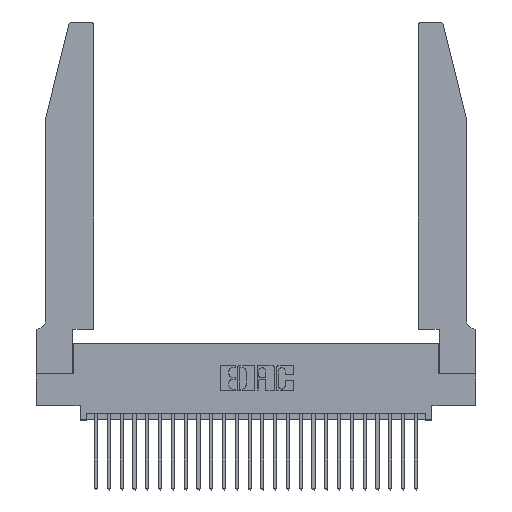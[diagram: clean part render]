
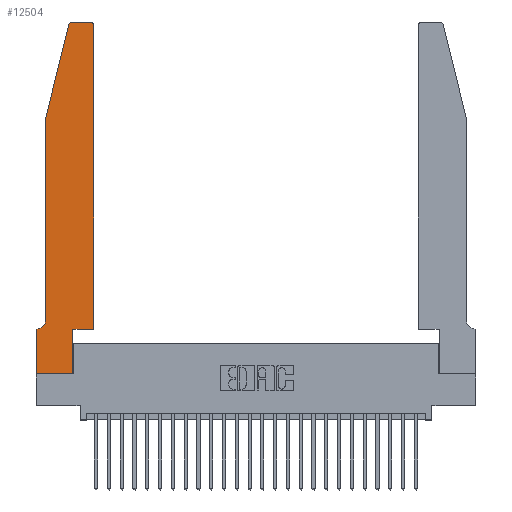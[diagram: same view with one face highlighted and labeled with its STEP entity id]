
A CAD part, top view. The second image highlights one B-rep face of the part: STEP entity #12504.
In plain terms, the highlighted planar face has unit normal (0, 0, 1).
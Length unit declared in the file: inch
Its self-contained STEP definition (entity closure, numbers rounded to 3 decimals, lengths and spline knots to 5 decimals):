
#205 = DIRECTION ( 'NONE',  ( 1., 0., 0. ) ) ;
#314 = ORIENTED_EDGE ( 'NONE', *, *, #13325, .T. ) ;
#342 = CARTESIAN_POINT ( 'NONE',  ( 0.284, 2.75, 0.37 ) ) ;
#738 = DIRECTION ( 'NONE',  ( 1., 0., 0. ) ) ;
#1029 = CARTESIAN_POINT ( 'NONE',  ( 0.25487, 2.72718, 0.37 ) ) ;
#1056 = CARTESIAN_POINT ( 'NONE',  ( 0.4205, 2.72, 0.37 ) ) ;
#1068 = VECTOR ( 'NONE', #16435, 39.37008 ) ;
#1119 = EDGE_CURVE ( 'NONE', #14258, #14778, #4081, .T. ) ;
#1410 = CARTESIAN_POINT ( 'NONE',  ( 0., 0., 0.37 ) ) ;
#1441 = LINE ( 'NONE', #9090, #6579 ) ;
#1597 = VECTOR ( 'NONE', #4198, 39.37008 ) ;
#1610 = LINE ( 'NONE', #23052, #12363 ) ;
#2075 = DIRECTION ( 'NONE',  ( 1., 0., 0. ) ) ;
#3099 = AXIS2_PLACEMENT_3D ( 'NONE', #27388, #14847, #2075 ) ;
#3253 = DIRECTION ( 'NONE',  ( 1., 0., 0. ) ) ;
#3386 = VECTOR ( 'NONE', #16997, 39.37008 ) ;
#3695 = VERTEX_POINT ( 'NONE', #342 ) ;
#3972 = CARTESIAN_POINT ( 'NONE',  ( 0.4505, 0.35, 0.37 ) ) ;
#4081 = LINE ( 'NONE', #23432, #3386 ) ;
#4198 = DIRECTION ( 'NONE',  ( -1., 0., 0. ) ) ;
#4357 = VERTEX_POINT ( 'NONE', #17513 ) ;
#4765 = VECTOR ( 'NONE', #12506, 39.37008 ) ;
#5065 = DIRECTION ( 'NONE',  ( 0., 0., -1. ) ) ;
#5778 = VECTOR ( 'NONE', #10602, 39.37008 ) ;
#5875 = FACE_OUTER_BOUND ( 'NONE', #19694, .T. ) ;
#5884 = ORIENTED_EDGE ( 'NONE', *, *, #19129, .T. ) ;
#6172 = EDGE_CURVE ( 'NONE', #13839, #14258, #1441, .T. ) ;
#6208 = AXIS2_PLACEMENT_3D ( 'NONE', #1056, #16011, #3253 ) ;
#6437 = CARTESIAN_POINT ( 'NONE',  ( 0.2865, 0.35, 0.37 ) ) ;
#6579 = VECTOR ( 'NONE', #15410, 39.37008 ) ;
#6647 = DIRECTION ( 'NONE',  ( 0., 1., 0. ) ) ;
#6660 = CARTESIAN_POINT ( 'NONE',  ( 0.0755, 2., 0.37 ) ) ;
#6893 = LINE ( 'NONE', #1410, #1068 ) ;
#7724 = ORIENTED_EDGE ( 'NONE', *, *, #6172, .T. ) ;
#8685 = EDGE_CURVE ( 'NONE', #4357, #13031, #1610, .T. ) ;
#9027 = LINE ( 'NONE', #3972, #19494 ) ;
#9090 = CARTESIAN_POINT ( 'NONE',  ( 0.0755, 2., 0.37 ) ) ;
#9771 = EDGE_CURVE ( 'NONE', #3695, #13839, #20169, .T. ) ;
#9810 = ORIENTED_EDGE ( 'NONE', *, *, #26122, .T. ) ;
#10602 = DIRECTION ( 'NONE',  ( -1., 0., 0. ) ) ;
#10643 = CARTESIAN_POINT ( 'NONE',  ( 0., 0.35, 0.37 ) ) ;
#11030 = ORIENTED_EDGE ( 'NONE', *, *, #17506, .T. ) ;
#11742 = EDGE_CURVE ( 'NONE', #14778, #12065, #23650, .T. ) ;
#12009 = EDGE_CURVE ( 'NONE', #13031, #23564, #17102, .T. ) ;
#12065 = VERTEX_POINT ( 'NONE', #17816 ) ;
#12188 = VECTOR ( 'NONE', #738, 39.37008 ) ;
#12207 = EDGE_CURVE ( 'NONE', #18627, #4357, #6893, .T. ) ;
#12313 = CARTESIAN_POINT ( 'NONE',  ( 0.4205, 2.75, 0.37 ) ) ;
#12363 = VECTOR ( 'NONE', #25150, 39.37008 ) ;
#12504 = ADVANCED_FACE ( 'NONE', ( #5875 ), #17228, .T. ) ;
#12506 = DIRECTION ( 'NONE',  ( 0., -1., 0. ) ) ;
#12954 = ORIENTED_EDGE ( 'NONE', *, *, #1119, .T. ) ;
#13031 = VERTEX_POINT ( 'NONE', #6437 ) ;
#13033 = CARTESIAN_POINT ( 'NONE',  ( 0., 0., 0.37 ) ) ;
#13067 = AXIS2_PLACEMENT_3D ( 'NONE', #25637, #13104, #205 ) ;
#13104 = DIRECTION ( 'NONE',  ( 0., 0., 1. ) ) ;
#13325 = EDGE_CURVE ( 'NONE', #18526, #26682, #24911, .T. ) ;
#13839 = VERTEX_POINT ( 'NONE', #1029 ) ;
#14258 = VERTEX_POINT ( 'NONE', #6660 ) ;
#14768 = CARTESIAN_POINT ( 'NONE',  ( 0.4505, 2.72, 0.37 ) ) ;
#14778 = VERTEX_POINT ( 'NONE', #18852 ) ;
#14847 = DIRECTION ( 'NONE',  ( 0., 0., 1. ) ) ;
#15105 = ORIENTED_EDGE ( 'NONE', *, *, #12207, .T. ) ;
#15410 = DIRECTION ( 'NONE',  ( -0.239, -0.971, 0. ) ) ;
#16011 = DIRECTION ( 'NONE',  ( 0., 0., 1. ) ) ;
#16115 = VERTEX_POINT ( 'NONE', #10643 ) ;
#16124 = CARTESIAN_POINT ( 'NONE',  ( 0.4505, 0.35, 0.37 ) ) ;
#16435 = DIRECTION ( 'NONE',  ( 1., 0., 0. ) ) ;
#16997 = DIRECTION ( 'NONE',  ( 0., -1., 0. ) ) ;
#16998 = LINE ( 'NONE', #25300, #5778 ) ;
#17102 = LINE ( 'NONE', #24031, #12188 ) ;
#17228 = PLANE ( 'NONE',  #13067 ) ;
#17506 = EDGE_CURVE ( 'NONE', #26682, #3695, #24779, .T. ) ;
#17513 = CARTESIAN_POINT ( 'NONE',  ( 0.2865, 0., 0.37 ) ) ;
#17545 = AXIS2_PLACEMENT_3D ( 'NONE', #17713, #5065, #19802 ) ;
#17713 = CARTESIAN_POINT ( 'NONE',  ( 0.0055, 0.42, 0.37 ) ) ;
#17816 = CARTESIAN_POINT ( 'NONE',  ( 0.0055, 0.35, 0.37 ) ) ;
#18526 = VERTEX_POINT ( 'NONE', #14768 ) ;
#18627 = VERTEX_POINT ( 'NONE', #13033 ) ;
#18852 = CARTESIAN_POINT ( 'NONE',  ( 0.0755, 0.42, 0.37 ) ) ;
#19129 = EDGE_CURVE ( 'NONE', #23564, #18526, #9027, .T. ) ;
#19494 = VECTOR ( 'NONE', #6647, 39.37008 ) ;
#19587 = ORIENTED_EDGE ( 'NONE', *, *, #26225, .T. ) ;
#19694 = EDGE_LOOP ( 'NONE', ( #11030, #26612, #7724, #12954, #21826, #19587, #9810, #15105, #21337, #26093, #5884, #314 ) ) ;
#19802 = DIRECTION ( 'NONE',  ( -1., 0., 0. ) ) ;
#20169 = CIRCLE ( 'NONE', #3099, 0.03 ) ;
#21337 = ORIENTED_EDGE ( 'NONE', *, *, #8685, .T. ) ;
#21826 = ORIENTED_EDGE ( 'NONE', *, *, #11742, .T. ) ;
#22927 = CARTESIAN_POINT ( 'NONE',  ( 0., 0., 0.37 ) ) ;
#23052 = CARTESIAN_POINT ( 'NONE',  ( 0.2865, 0.35, 0.37 ) ) ;
#23187 = CARTESIAN_POINT ( 'NONE',  ( 0.2605, 2.75, 0.37 ) ) ;
#23432 = CARTESIAN_POINT ( 'NONE',  ( 0.0755, 2., 0.37 ) ) ;
#23564 = VERTEX_POINT ( 'NONE', #16124 ) ;
#23650 = CIRCLE ( 'NONE', #17545, 0.07 ) ;
#24031 = CARTESIAN_POINT ( 'NONE',  ( 0.4505, 0.35, 0.37 ) ) ;
#24779 = LINE ( 'NONE', #23187, #1597 ) ;
#24911 = CIRCLE ( 'NONE', #6208, 0.03 ) ;
#25150 = DIRECTION ( 'NONE',  ( 0., 1., 0. ) ) ;
#25300 = CARTESIAN_POINT ( 'NONE',  ( 0.0755, 0.35, 0.37 ) ) ;
#25637 = CARTESIAN_POINT ( 'NONE',  ( 0., 0.35, 0.37 ) ) ;
#26093 = ORIENTED_EDGE ( 'NONE', *, *, #12009, .T. ) ;
#26122 = EDGE_CURVE ( 'NONE', #16115, #18627, #27143, .T. ) ;
#26225 = EDGE_CURVE ( 'NONE', #12065, #16115, #16998, .T. ) ;
#26612 = ORIENTED_EDGE ( 'NONE', *, *, #9771, .T. ) ;
#26682 = VERTEX_POINT ( 'NONE', #12313 ) ;
#27143 = LINE ( 'NONE', #22927, #4765 ) ;
#27388 = CARTESIAN_POINT ( 'NONE',  ( 0.284, 2.72, 0.37 ) ) ;
